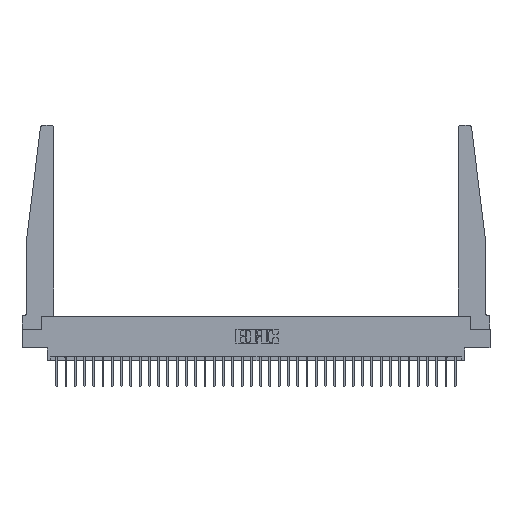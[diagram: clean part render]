
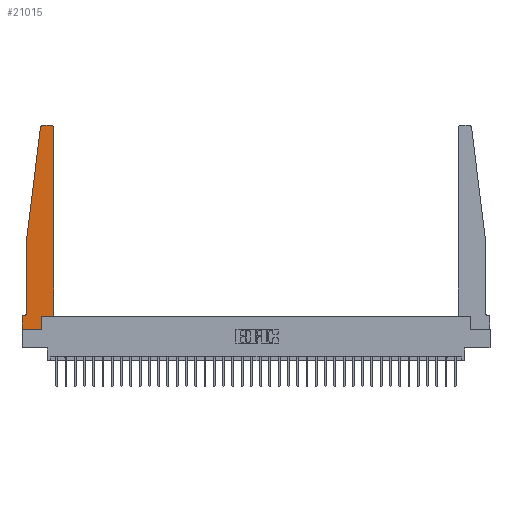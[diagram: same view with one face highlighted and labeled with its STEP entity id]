
A CAD part, top view. The second image highlights one B-rep face of the part: STEP entity #21015.
In plain terms, the highlighted planar face has unit normal (0, 0, 1).
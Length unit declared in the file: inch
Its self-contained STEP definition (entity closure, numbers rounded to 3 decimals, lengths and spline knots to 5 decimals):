
#30 = CARTESIAN_POINT ( 'NONE',  ( 0.015, 0.1875, 0.37 ) ) ;
#340 = CIRCLE ( 'NONE', #12357, 0.05 ) ;
#629 = CARTESIAN_POINT ( 'NONE',  ( 0.065, 0.1875, 0.37 ) ) ;
#688 = FACE_OUTER_BOUND ( 'NONE', #32383, .T. ) ;
#1085 = CIRCLE ( 'NONE', #17466, 0.03 ) ;
#2963 = VERTEX_POINT ( 'NONE', #30496 ) ;
#3033 = ORIENTED_EDGE ( 'NONE', *, *, #17884, .T. ) ;
#3073 = VECTOR ( 'NONE', #13489, 39.37008 ) ;
#3510 = CARTESIAN_POINT ( 'NONE',  ( 0.425, 2.72, 0.37 ) ) ;
#3563 = CARTESIAN_POINT ( 'NONE',  ( 0.2605, 0.18, 0.37 ) ) ;
#3566 = ORIENTED_EDGE ( 'NONE', *, *, #6322, .T. ) ;
#3732 = DIRECTION ( 'NONE',  ( 0., 1., 0. ) ) ;
#3743 = EDGE_CURVE ( 'NONE', #25455, #8828, #30085, .T. ) ;
#4060 = DIRECTION ( 'NONE',  ( 0., 0., 1. ) ) ;
#4978 = EDGE_CURVE ( 'NONE', #27203, #26903, #8014, .T. ) ;
#5117 = DIRECTION ( 'NONE',  ( -1., 0., 0. ) ) ;
#5154 = EDGE_CURVE ( 'NONE', #12375, #22617, #18229, .T. ) ;
#5470 = CARTESIAN_POINT ( 'NONE',  ( 0., 0.1875, 0.37 ) ) ;
#5505 = ORIENTED_EDGE ( 'NONE', *, *, #24310, .T. ) ;
#5711 = LINE ( 'NONE', #26606, #32815 ) ;
#6211 = CARTESIAN_POINT ( 'NONE',  ( 0.2605, 0.18, 0.37 ) ) ;
#6288 = DIRECTION ( 'NONE',  ( -0.122, -0.992, 0. ) ) ;
#6322 = EDGE_CURVE ( 'NONE', #13248, #7283, #16563, .T. ) ;
#6786 = CARTESIAN_POINT ( 'NONE',  ( 0.395, 2.72, 0.37 ) ) ;
#6896 = VECTOR ( 'NONE', #6288, 39.37008 ) ;
#7038 = AXIS2_PLACEMENT_3D ( 'NONE', #5470, #29098, #26866 ) ;
#7100 = ORIENTED_EDGE ( 'NONE', *, *, #7884, .T. ) ;
#7283 = VERTEX_POINT ( 'NONE', #6211 ) ;
#7341 = LINE ( 'NONE', #17431, #30511 ) ;
#7522 = CARTESIAN_POINT ( 'NONE',  ( 0.015, 0.2375, 0.37 ) ) ;
#7884 = EDGE_CURVE ( 'NONE', #2963, #19135, #340, .T. ) ;
#8014 = LINE ( 'NONE', #32314, #23097 ) ;
#8096 = EDGE_CURVE ( 'NONE', #8828, #2963, #13151, .T. ) ;
#8828 = VERTEX_POINT ( 'NONE', #17161 ) ;
#9336 = CARTESIAN_POINT ( 'NONE',  ( 0.27653, 2.75, 0.37 ) ) ;
#10422 = ORIENTED_EDGE ( 'NONE', *, *, #33673, .T. ) ;
#10834 = ORIENTED_EDGE ( 'NONE', *, *, #3743, .T. ) ;
#10849 = ORIENTED_EDGE ( 'NONE', *, *, #5154, .T. ) ;
#11632 = DIRECTION ( 'NONE',  ( 0., 0., 1. ) ) ;
#12357 = AXIS2_PLACEMENT_3D ( 'NONE', #7522, #33540, #5117 ) ;
#12375 = VERTEX_POINT ( 'NONE', #31481 ) ;
#13151 = LINE ( 'NONE', #21017, #3073 ) ;
#13248 = VERTEX_POINT ( 'NONE', #21228 ) ;
#13489 = DIRECTION ( 'NONE',  ( 0., -1., 0. ) ) ;
#13706 = VECTOR ( 'NONE', #29376, 39.37008 ) ;
#13768 = CARTESIAN_POINT ( 'NONE',  ( 0., 0., 0.37 ) ) ;
#14016 = VECTOR ( 'NONE', #3732, 39.37008 ) ;
#14229 = EDGE_CURVE ( 'NONE', #19135, #28890, #32288, .T. ) ;
#14550 = EDGE_CURVE ( 'NONE', #28890, #17440, #5711, .T. ) ;
#14996 = DIRECTION ( 'NONE',  ( -1., 0., 0. ) ) ;
#15451 = CARTESIAN_POINT ( 'NONE',  ( 0.425, 0.18, 0.37 ) ) ;
#16086 = ORIENTED_EDGE ( 'NONE', *, *, #4978, .T. ) ;
#16494 = VECTOR ( 'NONE', #22132, 39.37008 ) ;
#16563 = LINE ( 'NONE', #3563, #14016 ) ;
#17161 = CARTESIAN_POINT ( 'NONE',  ( 0.065, 1.25, 0.37 ) ) ;
#17431 = CARTESIAN_POINT ( 'NONE',  ( 0.425, 0.18, 0.37 ) ) ;
#17440 = VERTEX_POINT ( 'NONE', #13768 ) ;
#17466 = AXIS2_PLACEMENT_3D ( 'NONE', #6786, #4060, #30082 ) ;
#17884 = EDGE_CURVE ( 'NONE', #22617, #25455, #22019, .T. ) ;
#17899 = CARTESIAN_POINT ( 'NONE',  ( 0.25, 2.75, 0.37 ) ) ;
#18229 = LINE ( 'NONE', #17899, #26360 ) ;
#19052 = CARTESIAN_POINT ( 'NONE',  ( 0.24675, 2.72367, 0.37 ) ) ;
#19135 = VERTEX_POINT ( 'NONE', #30 ) ;
#19500 = CARTESIAN_POINT ( 'NONE',  ( 0.27653, 2.72, 0.37 ) ) ;
#20213 = CARTESIAN_POINT ( 'NONE',  ( 0., 0.1875, 0.37 ) ) ;
#20501 = DIRECTION ( 'NONE',  ( 1., 0., 0. ) ) ;
#21015 = ADVANCED_FACE ( 'NONE', ( #688 ), #32348, .T. ) ;
#21017 = CARTESIAN_POINT ( 'NONE',  ( 0.065, 1.25, 0.37 ) ) ;
#21228 = CARTESIAN_POINT ( 'NONE',  ( 0.2605, 0., 0.37 ) ) ;
#21644 = EDGE_CURVE ( 'NONE', #26903, #12375, #1085, .T. ) ;
#22019 = CIRCLE ( 'NONE', #28570, 0.03 ) ;
#22132 = DIRECTION ( 'NONE',  ( 1., 0., 0. ) ) ;
#22617 = VERTEX_POINT ( 'NONE', #9336 ) ;
#23097 = VECTOR ( 'NONE', #24423, 39.37008 ) ;
#23339 = DIRECTION ( 'NONE',  ( 0., -1., 0. ) ) ;
#24310 = EDGE_CURVE ( 'NONE', #17440, #13248, #24874, .T. ) ;
#24423 = DIRECTION ( 'NONE',  ( 0., 1., 0. ) ) ;
#24874 = LINE ( 'NONE', #32605, #16494 ) ;
#25228 = ORIENTED_EDGE ( 'NONE', *, *, #8096, .T. ) ;
#25455 = VERTEX_POINT ( 'NONE', #19052 ) ;
#26360 = VECTOR ( 'NONE', #14996, 39.37008 ) ;
#26606 = CARTESIAN_POINT ( 'NONE',  ( 0., 0., 0.37 ) ) ;
#26866 = DIRECTION ( 'NONE',  ( 1., 0., 0. ) ) ;
#26903 = VERTEX_POINT ( 'NONE', #3510 ) ;
#27008 = CARTESIAN_POINT ( 'NONE',  ( 0.065, 1.25, 0.37 ) ) ;
#27203 = VERTEX_POINT ( 'NONE', #15451 ) ;
#28570 = AXIS2_PLACEMENT_3D ( 'NONE', #19500, #11632, #32694 ) ;
#28890 = VERTEX_POINT ( 'NONE', #20213 ) ;
#29098 = DIRECTION ( 'NONE',  ( 0., 0., 1. ) ) ;
#29376 = DIRECTION ( 'NONE',  ( -1., 0., 0. ) ) ;
#30082 = DIRECTION ( 'NONE',  ( 1., 0., 0. ) ) ;
#30085 = LINE ( 'NONE', #27008, #6896 ) ;
#30496 = CARTESIAN_POINT ( 'NONE',  ( 0.065, 0.2375, 0.37 ) ) ;
#30511 = VECTOR ( 'NONE', #20501, 39.37008 ) ;
#31398 = ORIENTED_EDGE ( 'NONE', *, *, #21644, .T. ) ;
#31481 = CARTESIAN_POINT ( 'NONE',  ( 0.395, 2.75, 0.37 ) ) ;
#31867 = ORIENTED_EDGE ( 'NONE', *, *, #14550, .T. ) ;
#32055 = ORIENTED_EDGE ( 'NONE', *, *, #14229, .T. ) ;
#32288 = LINE ( 'NONE', #629, #13706 ) ;
#32314 = CARTESIAN_POINT ( 'NONE',  ( 0.425, 0.18, 0.37 ) ) ;
#32348 = PLANE ( 'NONE',  #7038 ) ;
#32383 = EDGE_LOOP ( 'NONE', ( #10849, #3033, #10834, #25228, #7100, #32055, #31867, #5505, #3566, #10422, #16086, #31398 ) ) ;
#32605 = CARTESIAN_POINT ( 'NONE',  ( 0., 0., 0.37 ) ) ;
#32694 = DIRECTION ( 'NONE',  ( 1., 0., 0. ) ) ;
#32815 = VECTOR ( 'NONE', #23339, 39.37008 ) ;
#33540 = DIRECTION ( 'NONE',  ( 0., 0., -1. ) ) ;
#33673 = EDGE_CURVE ( 'NONE', #7283, #27203, #7341, .T. ) ;
